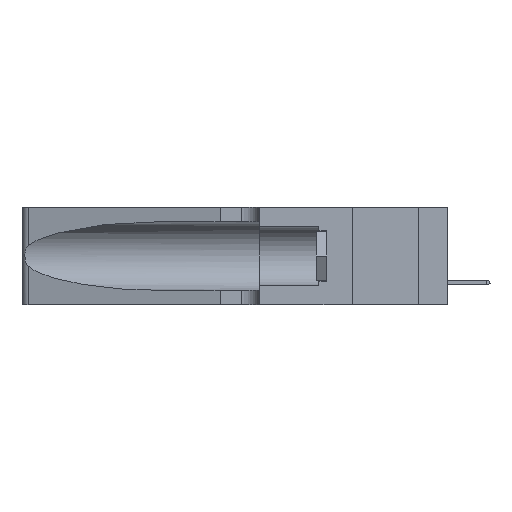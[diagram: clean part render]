
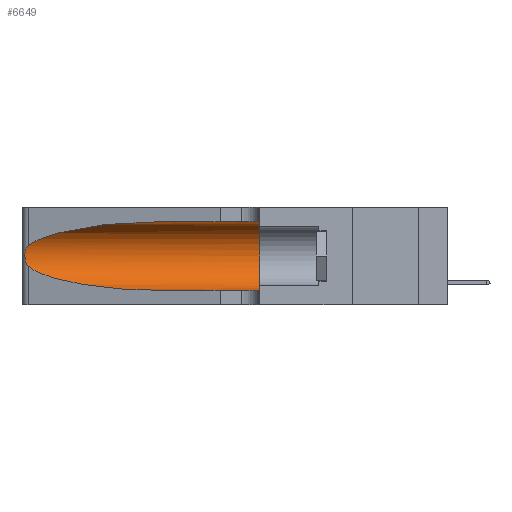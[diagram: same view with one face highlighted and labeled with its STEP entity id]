
A CAD part, left-side view. The second image highlights one B-rep face of the part: STEP entity #6649.
In plain terms, the highlighted cylindrical face has radius 3.308 mm (diameter 6.617 mm), a partial arc.
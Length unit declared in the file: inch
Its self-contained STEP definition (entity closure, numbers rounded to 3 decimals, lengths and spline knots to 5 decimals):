
#192 = CARTESIAN_POINT ( 'NONE',  ( 0.1305, 1.61858, 0.31525 ) ) ;
#289 = CARTESIAN_POINT ( 'NONE',  ( 0.1305, 0.72297, 0.31525 ) ) ;
#346 = ORIENTED_EDGE ( 'NONE', *, *, #18023, .T. ) ;
#976 = CARTESIAN_POINT ( 'NONE',  ( 0.1305, 1.61858, 0.185 ) ) ;
#1723 = DIRECTION ( 'NONE',  ( 0., 0., 1. ) ) ;
#2545 = CARTESIAN_POINT ( 'NONE',  ( 0.2373, 1.15595, 0.28018 ) ) ;
#4099 = DIRECTION ( 'NONE',  ( 0., -1., 0. ) ) ;
#4132 = LINE ( 'NONE', #16827, #14558 ) ;
#4247 = ORIENTED_EDGE ( 'NONE', *, *, #6709, .T. ) ;
#4520 = CARTESIAN_POINT ( 'NONE',  ( 0.25487, 1.22718, 0.22369 ) ) ;
#4758 = CARTESIAN_POINT ( 'NONE',  ( 0.1305, 0.35, 0.05475 ) ) ;
#4808 = AXIS2_PLACEMENT_3D ( 'NONE', #7898, #21419, #1723 ) ;
#5335 = VECTOR ( 'NONE', #4099, 39.37008 ) ;
#5470 = CARTESIAN_POINT ( 'NONE',  ( 0.26017, 1.23833, 0.17102 ) ) ;
#5518 = VERTEX_POINT ( 'NONE', #15082 ) ;
#5702 = B_SPLINE_CURVE_WITH_KNOTS ( 'NONE', 3,
 ( #6776, #9125, #13356, #17030, #24762, #21063, #7290, #17196, #5470, #23153, #19178, #11240, #24850, #13198 ),
 .UNSPECIFIED., .F., .F.,
 ( 4, 2, 2, 2, 2, 2, 4 ),
 ( 0., 0.00027, 0.00053, 0.00107, 0.0016, 0.00187, 0.00214 ),
 .UNSPECIFIED. ) ;
#6649 = ADVANCED_FACE ( 'NONE', ( #21679 ), #16465, .F. ) ;
#6709 = EDGE_CURVE ( 'NONE', #5518, #15368, #12937, .T. ) ;
#6776 = CARTESIAN_POINT ( 'NONE',  ( 0.25487, 1.22718, 0.22369 ) ) ;
#6982 = ORIENTED_EDGE ( 'NONE', *, *, #15675, .F. ) ;
#7290 = CARTESIAN_POINT ( 'NONE',  ( 0.26075, 1.23896, 0.19203 ) ) ;
#7898 = CARTESIAN_POINT ( 'NONE',  ( 0.1305, 0.35, 0.185 ) ) ;
#9125 = CARTESIAN_POINT ( 'NONE',  ( 0.25555, 1.22994, 0.2215 ) ) ;
#9964 =( BOUNDED_CURVE ( )  B_SPLINE_CURVE ( 3, ( #289, #19856, #2545, #4520 ),
 .UNSPECIFIED., .F., .T. ) 
 B_SPLINE_CURVE_WITH_KNOTS ( ( 4, 4 ),
 ( 1.5708, 2.84003 ),
 .UNSPECIFIED. ) 
 CURVE ( )  GEOMETRIC_REPRESENTATION_ITEM ( )  RATIONAL_B_SPLINE_CURVE ( ( 1., 0.87, 0.87, 1. ) ) 
 REPRESENTATION_ITEM ( '' )  );
#10201 = VERTEX_POINT ( 'NONE', #11585 ) ;
#10856 = EDGE_CURVE ( 'NONE', #15914, #5518, #5702, .T. ) ;
#11240 = CARTESIAN_POINT ( 'NONE',  ( 0.25639, 1.23186, 0.15144 ) ) ;
#11585 = CARTESIAN_POINT ( 'NONE',  ( 0.1305, 0.35, 0.31525 ) ) ;
#12267 = CARTESIAN_POINT ( 'NONE',  ( 0.1305, 0.72297, 0.05475 ) ) ;
#12937 =( BOUNDED_CURVE ( )  B_SPLINE_CURVE ( 3, ( #21194, #24983, #17079, #19065 ),
 .UNSPECIFIED., .F., .T. ) 
 B_SPLINE_CURVE_WITH_KNOTS ( ( 4, 4 ),
 ( 3.44316, 4.71239 ),
 .UNSPECIFIED. ) 
 CURVE ( )  GEOMETRIC_REPRESENTATION_ITEM ( )  RATIONAL_B_SPLINE_CURVE ( ( 1., 0.87, 0.87, 1. ) ) 
 REPRESENTATION_ITEM ( '' )  );
#13183 = CIRCLE ( 'NONE', #4808, 0.13025 ) ;
#13198 = CARTESIAN_POINT ( 'NONE',  ( 0.25487, 1.22718, 0.14631 ) ) ;
#13356 = CARTESIAN_POINT ( 'NONE',  ( 0.25639, 1.23184, 0.21858 ) ) ;
#13645 = LINE ( 'NONE', #192, #5335 ) ;
#14538 = AXIS2_PLACEMENT_3D ( 'NONE', #976, #24573, #14801 ) ;
#14558 = VECTOR ( 'NONE', #14798, 39.37008 ) ;
#14798 = DIRECTION ( 'NONE',  ( 0., -1., 0. ) ) ;
#14801 = DIRECTION ( 'NONE',  ( 0., 0., -1. ) ) ;
#15082 = CARTESIAN_POINT ( 'NONE',  ( 0.25487, 1.22718, 0.14631 ) ) ;
#15368 = VERTEX_POINT ( 'NONE', #12267 ) ;
#15675 = EDGE_CURVE ( 'NONE', #10201, #23247, #13183, .T. ) ;
#15914 = VERTEX_POINT ( 'NONE', #24071 ) ;
#16465 = CYLINDRICAL_SURFACE ( 'NONE', #14538, 0.13025 ) ;
#16827 = CARTESIAN_POINT ( 'NONE',  ( 0.1305, 1.61858, 0.05475 ) ) ;
#17030 = CARTESIAN_POINT ( 'NONE',  ( 0.25787, 1.23484, 0.2124 ) ) ;
#17079 = CARTESIAN_POINT ( 'NONE',  ( 0.18966, 0.96281, 0.05475 ) ) ;
#17196 = CARTESIAN_POINT ( 'NONE',  ( 0.26075, 1.23896, 0.178 ) ) ;
#17541 = ORIENTED_EDGE ( 'NONE', *, *, #20173, .F. ) ;
#18023 = EDGE_CURVE ( 'NONE', #19279, #15914, #9964, .T. ) ;
#18281 = CARTESIAN_POINT ( 'NONE',  ( 0.1305, 0.72297, 0.31525 ) ) ;
#19040 = ORIENTED_EDGE ( 'NONE', *, *, #10856, .T. ) ;
#19065 = CARTESIAN_POINT ( 'NONE',  ( 0.1305, 0.72297, 0.05475 ) ) ;
#19178 = CARTESIAN_POINT ( 'NONE',  ( 0.25789, 1.23486, 0.15765 ) ) ;
#19279 = VERTEX_POINT ( 'NONE', #18281 ) ;
#19856 = CARTESIAN_POINT ( 'NONE',  ( 0.18966, 0.96281, 0.31525 ) ) ;
#20044 = EDGE_CURVE ( 'NONE', #15368, #23247, #4132, .T. ) ;
#20173 = EDGE_CURVE ( 'NONE', #19279, #10201, #13645, .T. ) ;
#21063 = CARTESIAN_POINT ( 'NONE',  ( 0.26018, 1.23835, 0.19895 ) ) ;
#21194 = CARTESIAN_POINT ( 'NONE',  ( 0.25487, 1.22718, 0.14631 ) ) ;
#21330 = EDGE_LOOP ( 'NONE', ( #346, #19040, #4247, #22855, #6982, #17541 ) ) ;
#21419 = DIRECTION ( 'NONE',  ( 0., 1., 0. ) ) ;
#21679 = FACE_OUTER_BOUND ( 'NONE', #21330, .T. ) ;
#22855 = ORIENTED_EDGE ( 'NONE', *, *, #20044, .T. ) ;
#23153 = CARTESIAN_POINT ( 'NONE',  ( 0.25856, 1.23593, 0.16098 ) ) ;
#23247 = VERTEX_POINT ( 'NONE', #4758 ) ;
#24071 = CARTESIAN_POINT ( 'NONE',  ( 0.25487, 1.22718, 0.22369 ) ) ;
#24573 = DIRECTION ( 'NONE',  ( 0., -1., 0. ) ) ;
#24762 = CARTESIAN_POINT ( 'NONE',  ( 0.25854, 1.2359, 0.20912 ) ) ;
#24850 = CARTESIAN_POINT ( 'NONE',  ( 0.25555, 1.22993, 0.14849 ) ) ;
#24983 = CARTESIAN_POINT ( 'NONE',  ( 0.2373, 1.15595, 0.08982 ) ) ;
